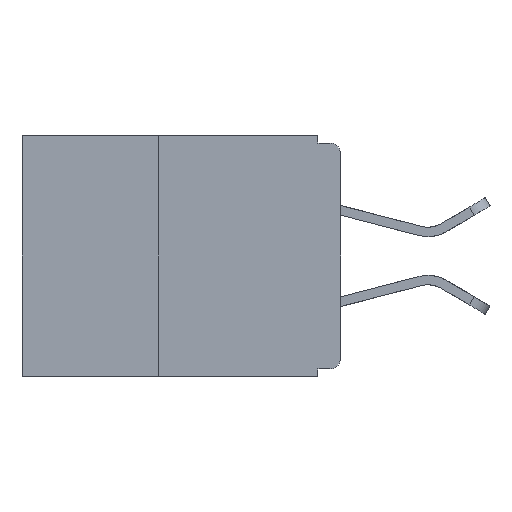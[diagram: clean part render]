
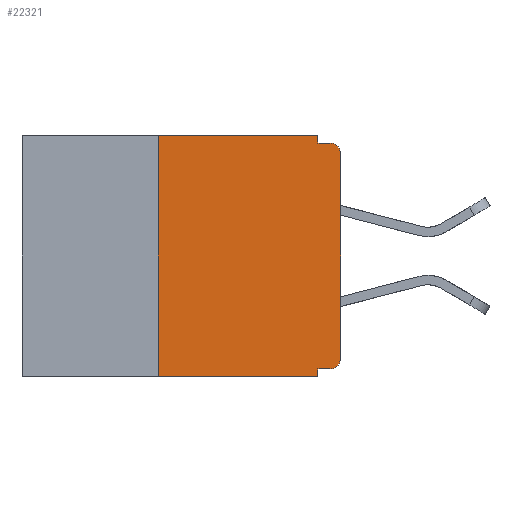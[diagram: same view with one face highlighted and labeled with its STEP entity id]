
A CAD part, left-side view. The second image highlights one B-rep face of the part: STEP entity #22321.
In plain terms, the highlighted planar face has unit normal (-1, 0, 0).
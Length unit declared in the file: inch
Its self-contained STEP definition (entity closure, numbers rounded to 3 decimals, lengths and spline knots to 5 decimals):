
#68 = PLANE ( 'NONE',  #4144 ) ;
#118 = FACE_OUTER_BOUND ( 'NONE', #20042, .T. ) ;
#292 = CARTESIAN_POINT ( 'NONE',  ( 0., 0.015, -0.305 ) ) ;
#396 = VERTEX_POINT ( 'NONE', #20986 ) ;
#409 = LINE ( 'NONE', #11695, #19753 ) ;
#625 = VECTOR ( 'NONE', #16713, 39.37008 ) ;
#1424 = CARTESIAN_POINT ( 'NONE',  ( 0., 0.25, -0.33 ) ) ;
#1770 = CARTESIAN_POINT ( 'NONE',  ( 0., 0.031, -0.01 ) ) ;
#2116 = CARTESIAN_POINT ( 'NONE',  ( 0., 0.437, 0. ) ) ;
#2322 = ORIENTED_EDGE ( 'NONE', *, *, #20397, .F. ) ;
#2336 = DIRECTION ( 'NONE',  ( 0., 0., -1. ) ) ;
#2404 = ORIENTED_EDGE ( 'NONE', *, *, #18453, .F. ) ;
#2470 = EDGE_CURVE ( 'NONE', #17374, #6128, #13656, .T. ) ;
#2479 = ORIENTED_EDGE ( 'NONE', *, *, #24161, .F. ) ;
#3511 = DIRECTION ( 'NONE',  ( 0., 0., 1. ) ) ;
#3612 = CARTESIAN_POINT ( 'NONE',  ( 0., 0.25, 0. ) ) ;
#4144 = AXIS2_PLACEMENT_3D ( 'NONE', #2116, #4210, #18091 ) ;
#4210 = DIRECTION ( 'NONE',  ( 1., 0., 0. ) ) ;
#4463 = ORIENTED_EDGE ( 'NONE', *, *, #16497, .F. ) ;
#4955 = CARTESIAN_POINT ( 'NONE',  ( 0., 0.437, 0. ) ) ;
#5979 = CARTESIAN_POINT ( 'NONE',  ( 0., 0., -0.025 ) ) ;
#6060 = LINE ( 'NONE', #14744, #625 ) ;
#6128 = VERTEX_POINT ( 'NONE', #11229 ) ;
#6163 = CARTESIAN_POINT ( 'NONE',  ( 0., 0., 0. ) ) ;
#6173 = CARTESIAN_POINT ( 'NONE',  ( 0., 0.031, 0. ) ) ;
#7484 = VERTEX_POINT ( 'NONE', #24491 ) ;
#7822 = LINE ( 'NONE', #13459, #17090 ) ;
#7934 = EDGE_CURVE ( 'NONE', #16902, #24430, #12150, .T. ) ;
#8166 = VERTEX_POINT ( 'NONE', #24610 ) ;
#8181 = DIRECTION ( 'NONE',  ( 0., 0., 1. ) ) ;
#8484 = DIRECTION ( 'NONE',  ( 0., 1., 0. ) ) ;
#8809 = VECTOR ( 'NONE', #16823, 39.37008 ) ;
#10498 = LINE ( 'NONE', #6163, #21995 ) ;
#11229 = CARTESIAN_POINT ( 'NONE',  ( 0., 0.015, -0.01 ) ) ;
#11345 = CARTESIAN_POINT ( 'NONE',  ( 0., 0.031, -0.33 ) ) ;
#11532 = VECTOR ( 'NONE', #8484, 39.37008 ) ;
#11536 = ORIENTED_EDGE ( 'NONE', *, *, #19155, .T. ) ;
#11695 = CARTESIAN_POINT ( 'NONE',  ( 0., 0., -0.01 ) ) ;
#12150 = LINE ( 'NONE', #18319, #11532 ) ;
#13459 = CARTESIAN_POINT ( 'NONE',  ( 0., 0.437, -0.33 ) ) ;
#13474 = VERTEX_POINT ( 'NONE', #6173 ) ;
#13656 = CIRCLE ( 'NONE', #21429, 0.015 ) ;
#13685 = DIRECTION ( 'NONE',  ( 0., -1., 0. ) ) ;
#14345 = DIRECTION ( 'NONE',  ( -1., 0., 0. ) ) ;
#14501 = CARTESIAN_POINT ( 'NONE',  ( 0., 0.015, -0.32 ) ) ;
#14561 = EDGE_CURVE ( 'NONE', #17310, #6128, #409, .T. ) ;
#14744 = CARTESIAN_POINT ( 'NONE',  ( 0., 0.031, 0. ) ) ;
#14948 = DIRECTION ( 'NONE',  ( 0., 0., -1. ) ) ;
#15413 = DIRECTION ( 'NONE',  ( 0., -1., 0. ) ) ;
#15958 = CIRCLE ( 'NONE', #16469, 0.015 ) ;
#16469 = AXIS2_PLACEMENT_3D ( 'NONE', #292, #14345, #2336 ) ;
#16497 = EDGE_CURVE ( 'NONE', #24430, #8166, #21689, .T. ) ;
#16608 = VECTOR ( 'NONE', #22907, 39.37008 ) ;
#16713 = DIRECTION ( 'NONE',  ( 0., 0., -1. ) ) ;
#16823 = DIRECTION ( 'NONE',  ( 0., -1., 0. ) ) ;
#16902 = VERTEX_POINT ( 'NONE', #14501 ) ;
#17090 = VECTOR ( 'NONE', #15413, 39.37008 ) ;
#17310 = VERTEX_POINT ( 'NONE', #1770 ) ;
#17374 = VERTEX_POINT ( 'NONE', #5979 ) ;
#17621 = LINE ( 'NONE', #1424, #22067 ) ;
#18091 = DIRECTION ( 'NONE',  ( 0., 0., -1. ) ) ;
#18319 = CARTESIAN_POINT ( 'NONE',  ( 0., 0., -0.32 ) ) ;
#18453 = EDGE_CURVE ( 'NONE', #20416, #13474, #18680, .T. ) ;
#18502 = DIRECTION ( 'NONE',  ( -1., 0., 0. ) ) ;
#18680 = LINE ( 'NONE', #4955, #8809 ) ;
#19112 = ORIENTED_EDGE ( 'NONE', *, *, #7934, .F. ) ;
#19155 = EDGE_CURVE ( 'NONE', #7484, #8166, #7822, .T. ) ;
#19539 = CARTESIAN_POINT ( 'NONE',  ( 0., 0.031, -0.32 ) ) ;
#19753 = VECTOR ( 'NONE', #13685, 39.37008 ) ;
#20042 = EDGE_LOOP ( 'NONE', ( #22651, #24398, #24421, #2479, #2404, #2322, #11536, #4463, #19112, #22615 ) ) ;
#20397 = EDGE_CURVE ( 'NONE', #7484, #20416, #17621, .T. ) ;
#20416 = VERTEX_POINT ( 'NONE', #3612 ) ;
#20986 = CARTESIAN_POINT ( 'NONE',  ( 0., 0., -0.305 ) ) ;
#21429 = AXIS2_PLACEMENT_3D ( 'NONE', #22765, #18502, #14948 ) ;
#21689 = LINE ( 'NONE', #11345, #16608 ) ;
#21995 = VECTOR ( 'NONE', #8181, 39.37008 ) ;
#22067 = VECTOR ( 'NONE', #3511, 39.37008 ) ;
#22321 = ADVANCED_FACE ( 'NONE', ( #118 ), #68, .F. ) ;
#22615 = ORIENTED_EDGE ( 'NONE', *, *, #25268, .T. ) ;
#22651 = ORIENTED_EDGE ( 'NONE', *, *, #23562, .T. ) ;
#22765 = CARTESIAN_POINT ( 'NONE',  ( 0., 0.015, -0.025 ) ) ;
#22907 = DIRECTION ( 'NONE',  ( 0., 0., -1. ) ) ;
#23562 = EDGE_CURVE ( 'NONE', #396, #17374, #10498, .T. ) ;
#24161 = EDGE_CURVE ( 'NONE', #13474, #17310, #6060, .T. ) ;
#24398 = ORIENTED_EDGE ( 'NONE', *, *, #2470, .T. ) ;
#24421 = ORIENTED_EDGE ( 'NONE', *, *, #14561, .F. ) ;
#24430 = VERTEX_POINT ( 'NONE', #19539 ) ;
#24491 = CARTESIAN_POINT ( 'NONE',  ( 0., 0.25, -0.33 ) ) ;
#24610 = CARTESIAN_POINT ( 'NONE',  ( 0., 0.031, -0.33 ) ) ;
#25268 = EDGE_CURVE ( 'NONE', #16902, #396, #15958, .T. ) ;
